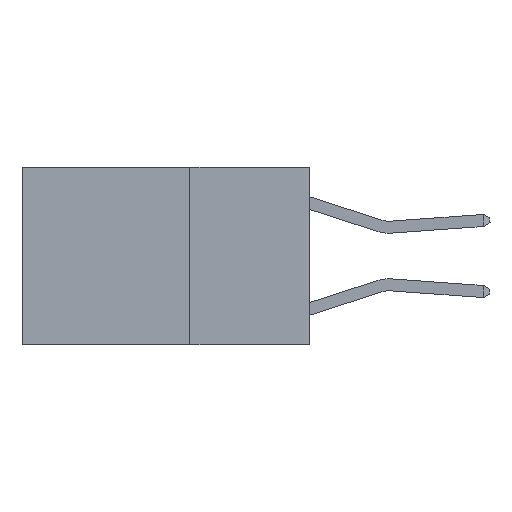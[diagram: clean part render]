
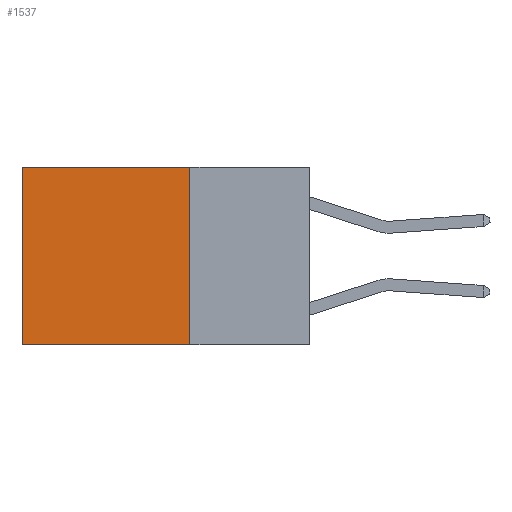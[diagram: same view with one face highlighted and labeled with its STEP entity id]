
A CAD part, left-side view. The second image highlights one B-rep face of the part: STEP entity #1537.
In plain terms, the highlighted planar face has unit normal (-1, 0, 0).
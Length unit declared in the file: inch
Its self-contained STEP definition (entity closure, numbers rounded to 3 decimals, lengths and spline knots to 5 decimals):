
#175 = CARTESIAN_POINT ( 'NONE',  ( 0.2625, 0.25, 0. ) ) ;
#207 = ORIENTED_EDGE ( 'NONE', *, *, #6977, .T. ) ;
#305 = CARTESIAN_POINT ( 'NONE',  ( 0.2625, 0.25, 0. ) ) ;
#417 = VECTOR ( 'NONE', #8575, 39.37008 ) ;
#636 = ORIENTED_EDGE ( 'NONE', *, *, #3822, .T. ) ;
#1015 = ORIENTED_EDGE ( 'NONE', *, *, #3274, .F. ) ;
#1370 = VERTEX_POINT ( 'NONE', #7514 ) ;
#1537 = ADVANCED_FACE ( 'NONE', ( #8382 ), #6964, .F. ) ;
#1740 = LINE ( 'NONE', #175, #4415 ) ;
#1807 = ORIENTED_EDGE ( 'NONE', *, *, #1871, .F. ) ;
#1870 = VECTOR ( 'NONE', #7690, 39.37008 ) ;
#1871 = EDGE_CURVE ( 'NONE', #2167, #5561, #4001, .T. ) ;
#2167 = VERTEX_POINT ( 'NONE', #8811 ) ;
#2571 = LINE ( 'NONE', #8857, #8560 ) ;
#3055 = AXIS2_PLACEMENT_3D ( 'NONE', #4766, #6923, #7795 ) ;
#3201 = DIRECTION ( 'NONE',  ( 0., 0., -1. ) ) ;
#3274 = EDGE_CURVE ( 'NONE', #1370, #2167, #1740, .T. ) ;
#3822 = EDGE_CURVE ( 'NONE', #1370, #5592, #5570, .T. ) ;
#3999 = CARTESIAN_POINT ( 'NONE',  ( 0.2625, 0.6, -0.37 ) ) ;
#4001 = LINE ( 'NONE', #7055, #1870 ) ;
#4415 = VECTOR ( 'NONE', #3201, 39.37008 ) ;
#4766 = CARTESIAN_POINT ( 'NONE',  ( 0.2625, 0.25, 0. ) ) ;
#5561 = VERTEX_POINT ( 'NONE', #3999 ) ;
#5570 = LINE ( 'NONE', #305, #417 ) ;
#5592 = VERTEX_POINT ( 'NONE', #9221 ) ;
#6505 = DIRECTION ( 'NONE',  ( 0., 0., -1. ) ) ;
#6923 = DIRECTION ( 'NONE',  ( 1., 0., 0. ) ) ;
#6964 = PLANE ( 'NONE',  #3055 ) ;
#6977 = EDGE_CURVE ( 'NONE', #5592, #5561, #2571, .T. ) ;
#7055 = CARTESIAN_POINT ( 'NONE',  ( 0.2625, 0.25, -0.37 ) ) ;
#7514 = CARTESIAN_POINT ( 'NONE',  ( 0.2625, 0.25, 0. ) ) ;
#7690 = DIRECTION ( 'NONE',  ( 0., 1., 0. ) ) ;
#7795 = DIRECTION ( 'NONE',  ( 0., 0., -1. ) ) ;
#8382 = FACE_OUTER_BOUND ( 'NONE', #8935, .T. ) ;
#8560 = VECTOR ( 'NONE', #6505, 39.37008 ) ;
#8575 = DIRECTION ( 'NONE',  ( 0., 1., 0. ) ) ;
#8811 = CARTESIAN_POINT ( 'NONE',  ( 0.2625, 0.25, -0.37 ) ) ;
#8857 = CARTESIAN_POINT ( 'NONE',  ( 0.2625, 0.6, 0. ) ) ;
#8935 = EDGE_LOOP ( 'NONE', ( #207, #1807, #1015, #636 ) ) ;
#9221 = CARTESIAN_POINT ( 'NONE',  ( 0.2625, 0.6, 0. ) ) ;
